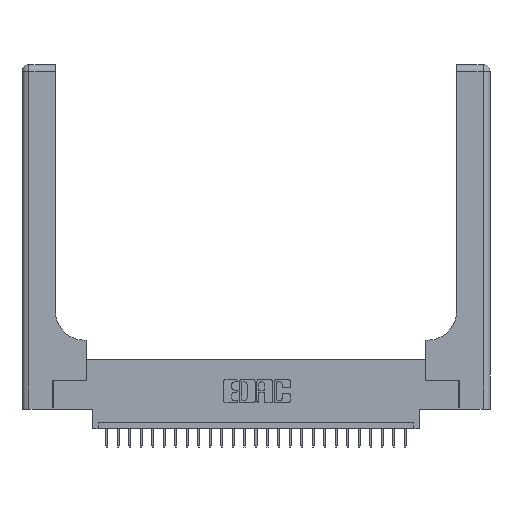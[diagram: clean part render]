
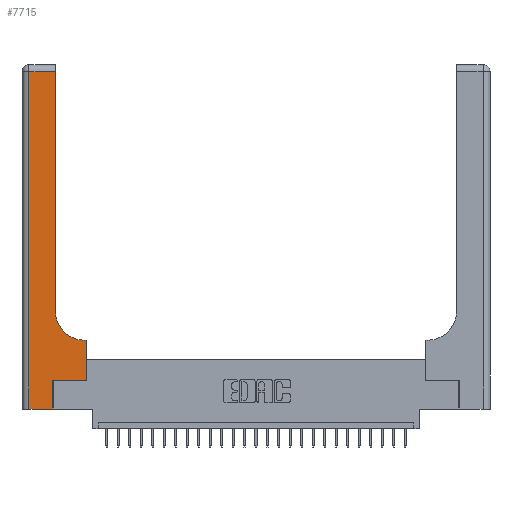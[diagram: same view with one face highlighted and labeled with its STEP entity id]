
A CAD part, top view. The second image highlights one B-rep face of the part: STEP entity #7715.
In plain terms, the highlighted planar face has unit normal (0, 0, 1).
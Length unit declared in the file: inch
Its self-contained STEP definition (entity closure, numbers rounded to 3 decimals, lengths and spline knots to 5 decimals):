
#150 = LINE ( 'NONE', #20797, #20584 ) ;
#231 = VERTEX_POINT ( 'NONE', #27401 ) ;
#775 = EDGE_LOOP ( 'NONE', ( #27567, #17151, #12934, #24576, #9590, #25341, #27091, #12123, #6287 ) ) ;
#920 = VERTEX_POINT ( 'NONE', #16407 ) ;
#1183 = FACE_OUTER_BOUND ( 'NONE', #775, .T. ) ;
#1336 = CARTESIAN_POINT ( 'NONE',  ( 0.5585, 0.6, 0.37 ) ) ;
#1766 = CARTESIAN_POINT ( 'NONE',  ( 0.2915, 3., 0.37 ) ) ;
#1950 = VECTOR ( 'NONE', #13910, 39.37008 ) ;
#2142 = DIRECTION ( 'NONE',  ( 0., 1., 0. ) ) ;
#2779 = VERTEX_POINT ( 'NONE', #17127 ) ;
#3094 = DIRECTION ( 'NONE',  ( -1., 0., 0. ) ) ;
#3486 = CARTESIAN_POINT ( 'NONE',  ( 0.06, 3., 0.37 ) ) ;
#3638 = CARTESIAN_POINT ( 'NONE',  ( 0.5415, 0.85, 0.37 ) ) ;
#3823 = CARTESIAN_POINT ( 'NONE',  ( 0.06, 0., 0.37 ) ) ;
#4034 = CARTESIAN_POINT ( 'NONE',  ( 0.269, 0.25, 0.37 ) ) ;
#4048 = LINE ( 'NONE', #1766, #26517 ) ;
#4199 = EDGE_CURVE ( 'NONE', #920, #20633, #150, .T. ) ;
#4258 = VERTEX_POINT ( 'NONE', #3823 ) ;
#4779 = LINE ( 'NONE', #10258, #9822 ) ;
#5635 = CARTESIAN_POINT ( 'NONE',  ( 0.5585, 0.25, 0.37 ) ) ;
#5816 = EDGE_CURVE ( 'NONE', #2779, #15313, #16114, .T. ) ;
#6023 = CARTESIAN_POINT ( 'NONE',  ( 0.06, 2.94, 0.37 ) ) ;
#6287 = ORIENTED_EDGE ( 'NONE', *, *, #8594, .T. ) ;
#6585 = CARTESIAN_POINT ( 'NONE',  ( 0.2915, 0.85, 0.37 ) ) ;
#7417 = VERTEX_POINT ( 'NONE', #1336 ) ;
#7547 = AXIS2_PLACEMENT_3D ( 'NONE', #3638, #22982, #27076 ) ;
#7715 = ADVANCED_FACE ( 'NONE', ( #1183 ), #10957, .F. ) ;
#8422 = DIRECTION ( 'NONE',  ( 0., 0., -1. ) ) ;
#8594 = EDGE_CURVE ( 'NONE', #231, #23394, #23638, .T. ) ;
#9015 = LINE ( 'NONE', #20340, #25767 ) ;
#9293 = EDGE_CURVE ( 'NONE', #24863, #2779, #4779, .T. ) ;
#9590 = ORIENTED_EDGE ( 'NONE', *, *, #9293, .T. ) ;
#9822 = VECTOR ( 'NONE', #18905, 39.37008 ) ;
#10044 = EDGE_CURVE ( 'NONE', #23394, #920, #4048, .T. ) ;
#10258 = CARTESIAN_POINT ( 'NONE',  ( 0.269, 0., 0.37 ) ) ;
#10957 = PLANE ( 'NONE',  #21558 ) ;
#11736 = EDGE_CURVE ( 'NONE', #4258, #24863, #27425, .T. ) ;
#12123 = ORIENTED_EDGE ( 'NONE', *, *, #21868, .T. ) ;
#12128 = DIRECTION ( 'NONE',  ( 0., -1., 0. ) ) ;
#12934 = ORIENTED_EDGE ( 'NONE', *, *, #18139, .T. ) ;
#13009 = DIRECTION ( 'NONE',  ( -1., 0., 0. ) ) ;
#13910 = DIRECTION ( 'NONE',  ( 1., 0., 0. ) ) ;
#14860 = CARTESIAN_POINT ( 'NONE',  ( 0., 3., 0.37 ) ) ;
#15313 = VERTEX_POINT ( 'NONE', #5635 ) ;
#15892 = CARTESIAN_POINT ( 'NONE',  ( 0., 0., 0.37 ) ) ;
#16114 = LINE ( 'NONE', #4034, #25836 ) ;
#16407 = CARTESIAN_POINT ( 'NONE',  ( 0.2915, 2.94, 0.37 ) ) ;
#16432 = EDGE_CURVE ( 'NONE', #15313, #7417, #21570, .T. ) ;
#16946 = CARTESIAN_POINT ( 'NONE',  ( 0.5585, 0.25, 0.37 ) ) ;
#17127 = CARTESIAN_POINT ( 'NONE',  ( 0.269, 0.25, 0.37 ) ) ;
#17151 = ORIENTED_EDGE ( 'NONE', *, *, #4199, .T. ) ;
#18139 = EDGE_CURVE ( 'NONE', #20633, #4258, #23216, .T. ) ;
#18727 = CARTESIAN_POINT ( 'NONE',  ( 0.269, 0., 0.37 ) ) ;
#18905 = DIRECTION ( 'NONE',  ( 0., 1., 0. ) ) ;
#20340 = CARTESIAN_POINT ( 'NONE',  ( 0.2915, 0.6, 0.37 ) ) ;
#20584 = VECTOR ( 'NONE', #20893, 39.37008 ) ;
#20633 = VERTEX_POINT ( 'NONE', #6023 ) ;
#20797 = CARTESIAN_POINT ( 'NONE',  ( 0., 2.94, 0.37 ) ) ;
#20883 = VECTOR ( 'NONE', #2142, 39.37008 ) ;
#20893 = DIRECTION ( 'NONE',  ( -1., 0., 0. ) ) ;
#21558 = AXIS2_PLACEMENT_3D ( 'NONE', #14860, #8422, #13009 ) ;
#21570 = LINE ( 'NONE', #16946, #20883 ) ;
#21868 = EDGE_CURVE ( 'NONE', #7417, #231, #9015, .T. ) ;
#22960 = DIRECTION ( 'NONE',  ( 0., 1., 0. ) ) ;
#22982 = DIRECTION ( 'NONE',  ( 0., 0., -1. ) ) ;
#23216 = LINE ( 'NONE', #3486, #27556 ) ;
#23394 = VERTEX_POINT ( 'NONE', #6585 ) ;
#23638 = CIRCLE ( 'NONE', #7547, 0.25 ) ;
#24576 = ORIENTED_EDGE ( 'NONE', *, *, #11736, .T. ) ;
#24863 = VERTEX_POINT ( 'NONE', #18727 ) ;
#25341 = ORIENTED_EDGE ( 'NONE', *, *, #5816, .T. ) ;
#25767 = VECTOR ( 'NONE', #3094, 39.37008 ) ;
#25836 = VECTOR ( 'NONE', #27477, 39.37008 ) ;
#26517 = VECTOR ( 'NONE', #22960, 39.37008 ) ;
#27076 = DIRECTION ( 'NONE',  ( 1., 0., 0. ) ) ;
#27091 = ORIENTED_EDGE ( 'NONE', *, *, #16432, .T. ) ;
#27401 = CARTESIAN_POINT ( 'NONE',  ( 0.5415, 0.6, 0.37 ) ) ;
#27425 = LINE ( 'NONE', #15892, #1950 ) ;
#27477 = DIRECTION ( 'NONE',  ( 1., 0., 0. ) ) ;
#27556 = VECTOR ( 'NONE', #12128, 39.37008 ) ;
#27567 = ORIENTED_EDGE ( 'NONE', *, *, #10044, .T. ) ;
